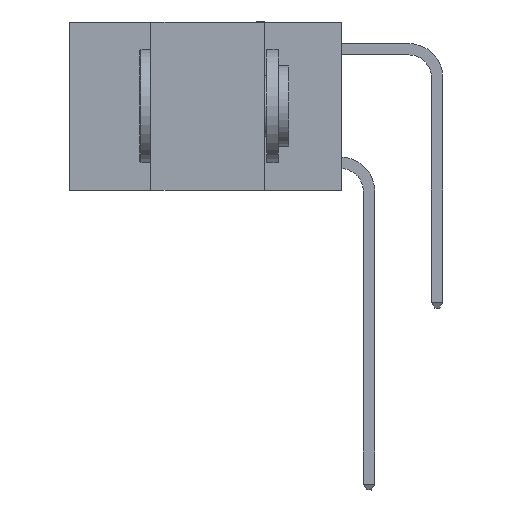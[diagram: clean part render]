
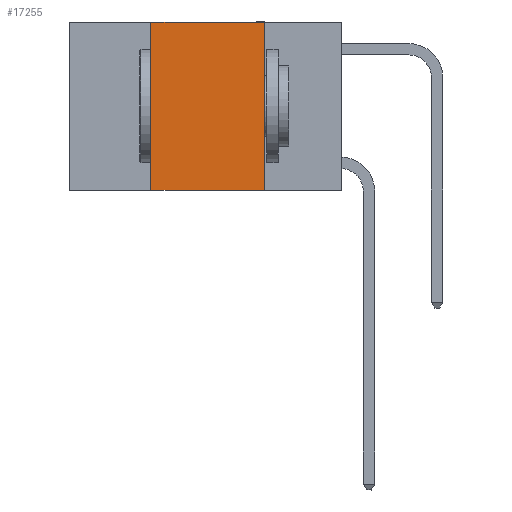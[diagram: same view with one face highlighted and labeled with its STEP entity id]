
A CAD part, left-side view. The second image highlights one B-rep face of the part: STEP entity #17255.
In plain terms, the highlighted planar face has unit normal (-1, 0, 0).
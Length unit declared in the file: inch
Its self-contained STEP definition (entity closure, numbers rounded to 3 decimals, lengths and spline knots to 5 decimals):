
#1882 = ORIENTED_EDGE ( 'NONE', *, *, #12228, .T. ) ;
#2068 = DIRECTION ( 'NONE',  ( 1., 0., 0. ) ) ;
#2519 = VECTOR ( 'NONE', #26938, 39.37008 ) ;
#5059 = CARTESIAN_POINT ( 'NONE',  ( 0., 0.42, 0. ) ) ;
#5561 = VECTOR ( 'NONE', #28100, 39.37008 ) ;
#5653 = EDGE_CURVE ( 'NONE', #8825, #26501, #8495, .T. ) ;
#5770 = VERTEX_POINT ( 'NONE', #22967 ) ;
#8144 = EDGE_CURVE ( 'NONE', #5770, #26308, #10103, .T. ) ;
#8390 = DIRECTION ( 'NONE',  ( 0., -1., 0. ) ) ;
#8495 = LINE ( 'NONE', #5059, #2519 ) ;
#8751 = AXIS2_PLACEMENT_3D ( 'NONE', #24007, #2068, #17644 ) ;
#8825 = VERTEX_POINT ( 'NONE', #12867 ) ;
#9296 = DIRECTION ( 'NONE',  ( 0., -1., 0. ) ) ;
#10103 = LINE ( 'NONE', #13004, #5561 ) ;
#10907 = ORIENTED_EDGE ( 'NONE', *, *, #5653, .F. ) ;
#11791 = EDGE_CURVE ( 'NONE', #26501, #5770, #12347, .T. ) ;
#12228 = EDGE_CURVE ( 'NONE', #8825, #26308, #24533, .T. ) ;
#12347 = LINE ( 'NONE', #13579, #23206 ) ;
#12413 = FACE_OUTER_BOUND ( 'NONE', #28345, .T. ) ;
#12867 = CARTESIAN_POINT ( 'NONE',  ( 0., 0.42, -0.37 ) ) ;
#13004 = CARTESIAN_POINT ( 'NONE',  ( 0., 0.17, 0. ) ) ;
#13579 = CARTESIAN_POINT ( 'NONE',  ( 0., 0.6, 0. ) ) ;
#17255 = ADVANCED_FACE ( 'NONE', ( #12413 ), #19674, .F. ) ;
#17630 = CARTESIAN_POINT ( 'NONE',  ( 0., 0.42, 0. ) ) ;
#17644 = DIRECTION ( 'NONE',  ( 0., 0., -1. ) ) ;
#18823 = VECTOR ( 'NONE', #8390, 39.37008 ) ;
#19336 = CARTESIAN_POINT ( 'NONE',  ( 0., 0.6, -0.37 ) ) ;
#19674 = PLANE ( 'NONE',  #8751 ) ;
#20231 = ORIENTED_EDGE ( 'NONE', *, *, #11791, .F. ) ;
#22967 = CARTESIAN_POINT ( 'NONE',  ( 0., 0.17, 0. ) ) ;
#23206 = VECTOR ( 'NONE', #9296, 39.37008 ) ;
#24007 = CARTESIAN_POINT ( 'NONE',  ( 0., 0.6, 0. ) ) ;
#24533 = LINE ( 'NONE', #19336, #18823 ) ;
#25497 = ORIENTED_EDGE ( 'NONE', *, *, #8144, .F. ) ;
#26308 = VERTEX_POINT ( 'NONE', #27862 ) ;
#26501 = VERTEX_POINT ( 'NONE', #17630 ) ;
#26938 = DIRECTION ( 'NONE',  ( 0., 0., 1. ) ) ;
#27862 = CARTESIAN_POINT ( 'NONE',  ( 0., 0.17, -0.37 ) ) ;
#28100 = DIRECTION ( 'NONE',  ( 0., 0., -1. ) ) ;
#28345 = EDGE_LOOP ( 'NONE', ( #25497, #20231, #10907, #1882 ) ) ;
